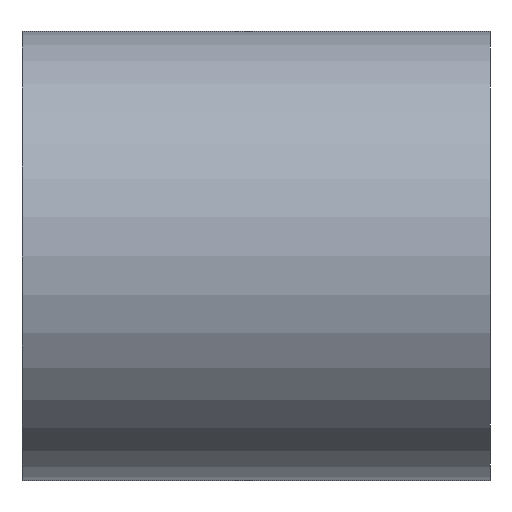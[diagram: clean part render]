
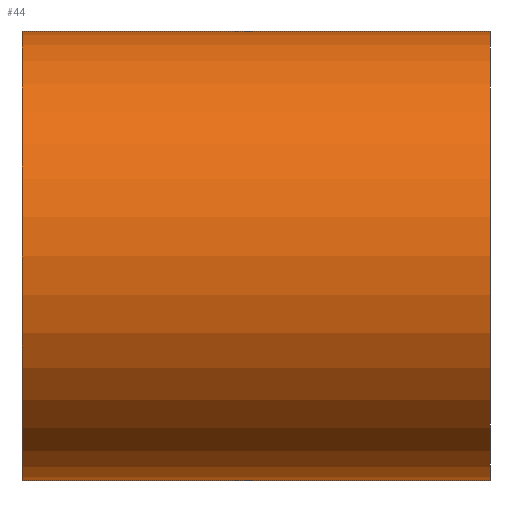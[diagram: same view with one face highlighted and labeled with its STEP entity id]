
A CAD part, front view. The second image highlights one B-rep face of the part: STEP entity #44.
In plain terms, the highlighted cylindrical face has radius 3.048 mm (diameter 6.096 mm), a partial arc.
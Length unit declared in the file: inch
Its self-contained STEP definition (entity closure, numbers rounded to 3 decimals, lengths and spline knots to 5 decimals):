
#10 = ORIENTED_EDGE ( 'NONE', *, *, #40, .F. ) ;
#12 = VERTEX_POINT ( 'NONE', #200 ) ;
#13 = CIRCLE ( 'NONE', #118, 0.12 ) ;
#20 = VERTEX_POINT ( 'NONE', #222 ) ;
#40 = EDGE_CURVE ( 'NONE', #41, #12, #119, .T. ) ;
#41 = VERTEX_POINT ( 'NONE', #204 ) ;
#44 = ADVANCED_FACE ( 'NONE', ( #100 ), #54, .T. ) ;
#46 = ORIENTED_EDGE ( 'NONE', *, *, #61, .T. ) ;
#50 = VERTEX_POINT ( 'NONE', #166 ) ;
#51 = EDGE_CURVE ( 'NONE', #20, #41, #13, .T. ) ;
#54 = CYLINDRICAL_SURFACE ( 'NONE', #216, 0.12 ) ;
#58 = ORIENTED_EDGE ( 'NONE', *, *, #104, .T. ) ;
#61 = EDGE_CURVE ( 'NONE', #50, #12, #105, .T. ) ;
#70 = EDGE_LOOP ( 'NONE', ( #10, #179, #58, #46 ) ) ;
#76 = DIRECTION ( 'NONE',  ( -1., 0., 0. ) ) ;
#77 = CARTESIAN_POINT ( 'NONE',  ( 0.25, 0., 0.12 ) ) ;
#82 = VECTOR ( 'NONE', #195, 39.37008 ) ;
#100 = FACE_OUTER_BOUND ( 'NONE', #70, .T. ) ;
#104 = EDGE_CURVE ( 'NONE', #20, #50, #161, .T. ) ;
#105 = CIRCLE ( 'NONE', #202, 0.12 ) ;
#118 = AXIS2_PLACEMENT_3D ( 'NONE', #148, #147, #140 ) ;
#119 = LINE ( 'NONE', #182, #82 ) ;
#122 = DIRECTION ( 'NONE',  ( 0., 0., -1. ) ) ;
#123 = DIRECTION ( 'NONE',  ( 1., 0., 0. ) ) ;
#125 = CARTESIAN_POINT ( 'NONE',  ( 0., 0., 0. ) ) ;
#140 = DIRECTION ( 'NONE',  ( 0., 0., -1. ) ) ;
#147 = DIRECTION ( 'NONE',  ( 1., 0., 0. ) ) ;
#148 = CARTESIAN_POINT ( 'NONE',  ( 0.25, 0., 0. ) ) ;
#151 = VECTOR ( 'NONE', #76, 39.37008 ) ;
#161 = LINE ( 'NONE', #77, #151 ) ;
#166 = CARTESIAN_POINT ( 'NONE',  ( 0., 0., 0.12 ) ) ;
#172 = DIRECTION ( 'NONE',  ( -1., 0., 0. ) ) ;
#173 = CARTESIAN_POINT ( 'NONE',  ( 0.25, 0., 0. ) ) ;
#179 = ORIENTED_EDGE ( 'NONE', *, *, #51, .F. ) ;
#182 = CARTESIAN_POINT ( 'NONE',  ( 0.25, 0., -0.12 ) ) ;
#186 = DIRECTION ( 'NONE',  ( 0., 0., 1. ) ) ;
#195 = DIRECTION ( 'NONE',  ( -1., 0., 0. ) ) ;
#200 = CARTESIAN_POINT ( 'NONE',  ( 0., 0., -0.12 ) ) ;
#202 = AXIS2_PLACEMENT_3D ( 'NONE', #125, #123, #122 ) ;
#204 = CARTESIAN_POINT ( 'NONE',  ( 0.25, 0., -0.12 ) ) ;
#216 = AXIS2_PLACEMENT_3D ( 'NONE', #173, #172, #186 ) ;
#222 = CARTESIAN_POINT ( 'NONE',  ( 0.25, 0., 0.12 ) ) ;
